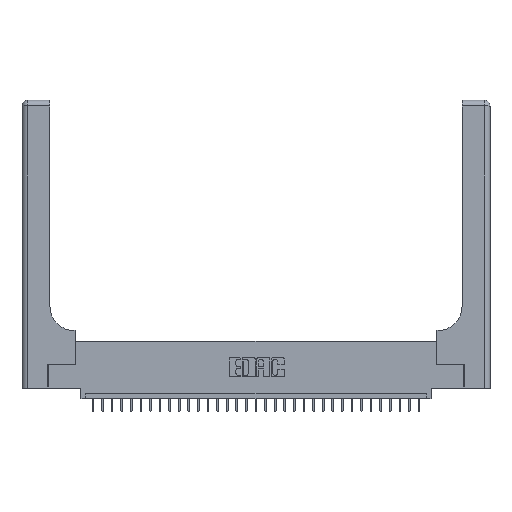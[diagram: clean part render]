
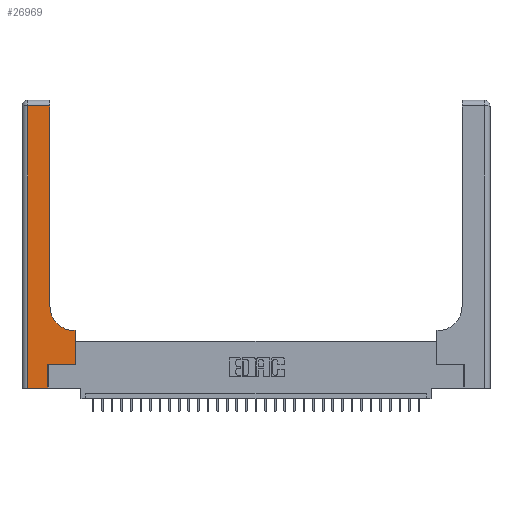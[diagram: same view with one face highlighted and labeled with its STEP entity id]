
A CAD part, top view. The second image highlights one B-rep face of the part: STEP entity #26969.
In plain terms, the highlighted planar face has unit normal (0, 0, 1).
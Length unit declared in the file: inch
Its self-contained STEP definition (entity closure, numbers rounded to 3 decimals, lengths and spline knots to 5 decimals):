
#148 = FACE_OUTER_BOUND ( 'NONE', #17652, .T. ) ;
#335 = CARTESIAN_POINT ( 'NONE',  ( 0.5585, 0.6, 0.37 ) ) ;
#714 = ORIENTED_EDGE ( 'NONE', *, *, #8620, .T. ) ;
#871 = LINE ( 'NONE', #10945, #16433 ) ;
#973 = VERTEX_POINT ( 'NONE', #22929 ) ;
#1387 = CARTESIAN_POINT ( 'NONE',  ( 0.5585, 0.25, 0.37 ) ) ;
#2858 = CARTESIAN_POINT ( 'NONE',  ( 0.5415, 0.6, 0.37 ) ) ;
#2929 = AXIS2_PLACEMENT_3D ( 'NONE', #15209, #15372, #23129 ) ;
#3270 = PLANE ( 'NONE',  #2929 ) ;
#3530 = LINE ( 'NONE', #1387, #7515 ) ;
#4688 = DIRECTION ( 'NONE',  ( 0., 1., 0. ) ) ;
#4706 = EDGE_CURVE ( 'NONE', #973, #27156, #21977, .T. ) ;
#4813 = VERTEX_POINT ( 'NONE', #25440 ) ;
#5360 = EDGE_CURVE ( 'NONE', #30273, #15692, #871, .T. ) ;
#5802 = ORIENTED_EDGE ( 'NONE', *, *, #21683, .T. ) ;
#6337 = DIRECTION ( 'NONE',  ( 0., 1., 0. ) ) ;
#7515 = VECTOR ( 'NONE', #6337, 39.37008 ) ;
#7522 = CARTESIAN_POINT ( 'NONE',  ( 0.5585, 0.25, 0.37 ) ) ;
#8620 = EDGE_CURVE ( 'NONE', #13865, #30273, #3530, .T. ) ;
#8720 = EDGE_CURVE ( 'NONE', #15692, #20050, #29147, .T. ) ;
#8798 = ORIENTED_EDGE ( 'NONE', *, *, #23320, .T. ) ;
#9092 = AXIS2_PLACEMENT_3D ( 'NONE', #9961, #14445, #12289 ) ;
#9366 = VECTOR ( 'NONE', #18319, 39.37008 ) ;
#9382 = DIRECTION ( 'NONE',  ( 1., 0., 0. ) ) ;
#9771 = DIRECTION ( 'NONE',  ( 0., -1., 0. ) ) ;
#9961 = CARTESIAN_POINT ( 'NONE',  ( 0.5415, 0.85, 0.37 ) ) ;
#10305 = EDGE_CURVE ( 'NONE', #4813, #973, #22515, .T. ) ;
#10388 = CARTESIAN_POINT ( 'NONE',  ( 0.2915, 0.85, 0.37 ) ) ;
#10672 = VERTEX_POINT ( 'NONE', #26919 ) ;
#10945 = CARTESIAN_POINT ( 'NONE',  ( 0.2915, 0.6, 0.37 ) ) ;
#12089 = CARTESIAN_POINT ( 'NONE',  ( 0.269, 0.25, 0.37 ) ) ;
#12289 = DIRECTION ( 'NONE',  ( 1., 0., 0. ) ) ;
#13865 = VERTEX_POINT ( 'NONE', #7522 ) ;
#14334 = CARTESIAN_POINT ( 'NONE',  ( 0.269, 0., 0.37 ) ) ;
#14445 = DIRECTION ( 'NONE',  ( 0., 0., -1. ) ) ;
#14882 = EDGE_CURVE ( 'NONE', #18841, #13865, #31191, .T. ) ;
#15209 = CARTESIAN_POINT ( 'NONE',  ( 0., 3., 0.37 ) ) ;
#15372 = DIRECTION ( 'NONE',  ( 0., 0., -1. ) ) ;
#15692 = VERTEX_POINT ( 'NONE', #2858 ) ;
#16433 = VECTOR ( 'NONE', #18728, 39.37008 ) ;
#17652 = EDGE_LOOP ( 'NONE', ( #8798, #18617, #26535, #20127, #5802, #29530, #714, #27610, #29240 ) ) ;
#18131 = EDGE_CURVE ( 'NONE', #10672, #4813, #20107, .T. ) ;
#18319 = DIRECTION ( 'NONE',  ( 1., 0., 0. ) ) ;
#18617 = ORIENTED_EDGE ( 'NONE', *, *, #18131, .T. ) ;
#18728 = DIRECTION ( 'NONE',  ( -1., 0., 0. ) ) ;
#18841 = VERTEX_POINT ( 'NONE', #12089 ) ;
#19594 = LINE ( 'NONE', #21746, #28706 ) ;
#20050 = VERTEX_POINT ( 'NONE', #10388 ) ;
#20107 = LINE ( 'NONE', #32507, #21600 ) ;
#20127 = ORIENTED_EDGE ( 'NONE', *, *, #4706, .T. ) ;
#20959 = CARTESIAN_POINT ( 'NONE',  ( 0.269, 0.25, 0.37 ) ) ;
#21472 = CARTESIAN_POINT ( 'NONE',  ( 0.269, 0., 0.37 ) ) ;
#21600 = VECTOR ( 'NONE', #27715, 39.37008 ) ;
#21683 = EDGE_CURVE ( 'NONE', #27156, #18841, #21785, .T. ) ;
#21746 = CARTESIAN_POINT ( 'NONE',  ( 0.2915, 3., 0.37 ) ) ;
#21785 = LINE ( 'NONE', #14334, #32331 ) ;
#21854 = VECTOR ( 'NONE', #9771, 39.37008 ) ;
#21977 = LINE ( 'NONE', #32037, #29032 ) ;
#22515 = LINE ( 'NONE', #26959, #21854 ) ;
#22929 = CARTESIAN_POINT ( 'NONE',  ( 0.06, 0., 0.37 ) ) ;
#23129 = DIRECTION ( 'NONE',  ( -1., 0., 0. ) ) ;
#23320 = EDGE_CURVE ( 'NONE', #20050, #10672, #19594, .T. ) ;
#24421 = DIRECTION ( 'NONE',  ( 0., 1., 0. ) ) ;
#25440 = CARTESIAN_POINT ( 'NONE',  ( 0.06, 2.94, 0.37 ) ) ;
#26535 = ORIENTED_EDGE ( 'NONE', *, *, #10305, .T. ) ;
#26919 = CARTESIAN_POINT ( 'NONE',  ( 0.2915, 2.94, 0.37 ) ) ;
#26959 = CARTESIAN_POINT ( 'NONE',  ( 0.06, 3., 0.37 ) ) ;
#26969 = ADVANCED_FACE ( 'NONE', ( #148 ), #3270, .F. ) ;
#27156 = VERTEX_POINT ( 'NONE', #21472 ) ;
#27610 = ORIENTED_EDGE ( 'NONE', *, *, #5360, .T. ) ;
#27715 = DIRECTION ( 'NONE',  ( -1., 0., 0. ) ) ;
#28706 = VECTOR ( 'NONE', #4688, 39.37008 ) ;
#29032 = VECTOR ( 'NONE', #9382, 39.37008 ) ;
#29147 = CIRCLE ( 'NONE', #9092, 0.25 ) ;
#29240 = ORIENTED_EDGE ( 'NONE', *, *, #8720, .T. ) ;
#29530 = ORIENTED_EDGE ( 'NONE', *, *, #14882, .T. ) ;
#30273 = VERTEX_POINT ( 'NONE', #335 ) ;
#31191 = LINE ( 'NONE', #20959, #9366 ) ;
#32037 = CARTESIAN_POINT ( 'NONE',  ( 0., 0., 0.37 ) ) ;
#32331 = VECTOR ( 'NONE', #24421, 39.37008 ) ;
#32507 = CARTESIAN_POINT ( 'NONE',  ( 0., 2.94, 0.37 ) ) ;
